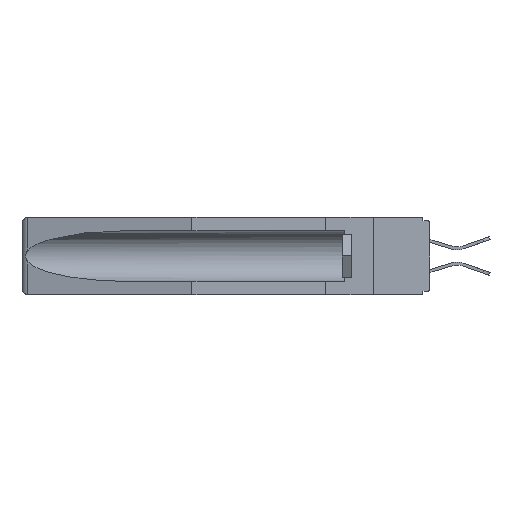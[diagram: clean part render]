
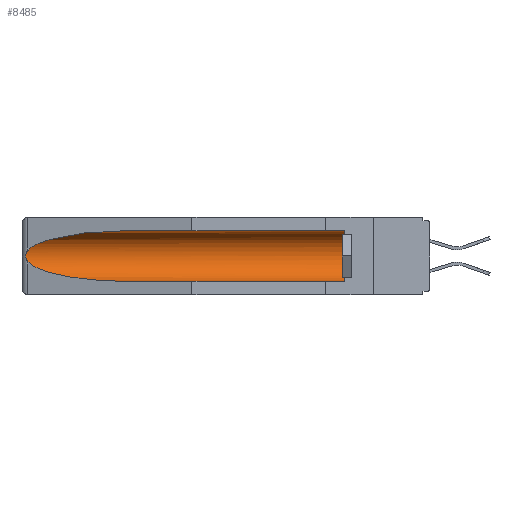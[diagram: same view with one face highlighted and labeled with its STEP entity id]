
A CAD part, left-side view. The second image highlights one B-rep face of the part: STEP entity #8485.
In plain terms, the highlighted cylindrical face has radius 2.857 mm (diameter 5.715 mm), a partial arc.
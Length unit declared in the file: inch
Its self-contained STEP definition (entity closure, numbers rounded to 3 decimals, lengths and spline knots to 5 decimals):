
#535 = AXIS2_PLACEMENT_3D ( 'NONE', #24284, #26498, #13403 ) ;
#593 = EDGE_CURVE ( 'NONE', #28294, #17367, #24356, .T. ) ;
#643 = EDGE_CURVE ( 'NONE', #16500, #28294, #3115, .T. ) ;
#1154 = CARTESIAN_POINT ( 'NONE',  ( 0.26537, 1.52718, -0.19328 ) ) ;
#2209 = CARTESIAN_POINT ( 'NONE',  ( 0.155, 1.07973, -0.059 ) ) ;
#3101 = VERTEX_POINT ( 'NONE', #14312 ) ;
#3115 = B_SPLINE_CURVE_WITH_KNOTS ( 'NONE', 3,
 ( #3253, #23229, #25435, #16695, #3615, #5355, #20636, #7530, #18514, #22962 ),
 .UNSPECIFIED., .F., .F.,
 ( 4, 2, 2, 2, 4 ),
 ( 0., 0.00029, 0.00058, 0.00087, 0.00117 ),
 .UNSPECIFIED. ) ;
#3253 = CARTESIAN_POINT ( 'NONE',  ( 0.26537, 1.52718, -0.14972 ) ) ;
#3615 = CARTESIAN_POINT ( 'NONE',  ( 0.2675, 1.53308, -0.16763 ) ) ;
#3891 = VERTEX_POINT ( 'NONE', #6112 ) ;
#5323 = AXIS2_PLACEMENT_3D ( 'NONE', #17474, #10945, #17375 ) ;
#5355 = CARTESIAN_POINT ( 'NONE',  ( 0.2675, 1.53308, -0.17534 ) ) ;
#5630 = CARTESIAN_POINT ( 'NONE',  ( 0.25451, 1.48313, -0.24835 ) ) ;
#6112 = CARTESIAN_POINT ( 'NONE',  ( 0.155, 1.07973, -0.059 ) ) ;
#6409 = ORIENTED_EDGE ( 'NONE', *, *, #643, .T. ) ;
#7530 = CARTESIAN_POINT ( 'NONE',  ( 0.26655, 1.53094, -0.18657 ) ) ;
#7807 = CARTESIAN_POINT ( 'NONE',  ( 0.21114, 1.30732, -0.284 ) ) ;
#7899 = CARTESIAN_POINT ( 'NONE',  ( 0.155, 1.07973, -0.284 ) ) ;
#8485 = ADVANCED_FACE ( 'NONE', ( #27992 ), #13875, .F. ) ;
#9525 = DIRECTION ( 'NONE',  ( 0., 1., 0. ) ) ;
#9707 = CARTESIAN_POINT ( 'NONE',  ( 0.26537, 1.52718, -0.14972 ) ) ;
#10874 = CARTESIAN_POINT ( 'NONE',  ( 0.155, 1.07973, -0.284 ) ) ;
#10945 = DIRECTION ( 'NONE',  ( 0., -1., 0. ) ) ;
#11147 =( BOUNDED_CURVE ( )  B_SPLINE_CURVE ( 3, ( #2209, #15069, #26049, #21698 ),
 .UNSPECIFIED., .F., .F. ) 
 B_SPLINE_CURVE_WITH_KNOTS ( ( 4, 4 ),
 ( 4.71239, 6.08839 ),
 .UNSPECIFIED. ) 
 CURVE ( )  GEOMETRIC_REPRESENTATION_ITEM ( )  RATIONAL_B_SPLINE_CURVE ( ( 1., 0.848, 0.848, 1. ) ) 
 REPRESENTATION_ITEM ( '' )  );
#11798 = DIRECTION ( 'NONE',  ( 0., 1., 0. ) ) ;
#13403 = DIRECTION ( 'NONE',  ( 0., 0., 1. ) ) ;
#13875 = CYLINDRICAL_SURFACE ( 'NONE', #535, 0.1125 ) ;
#14205 = EDGE_LOOP ( 'NONE', ( #18307, #6409, #16696, #26466, #26667, #27182 ) ) ;
#14312 = CARTESIAN_POINT ( 'NONE',  ( 0.155, 0.126, -0.284 ) ) ;
#15069 = CARTESIAN_POINT ( 'NONE',  ( 0.21114, 1.30732, -0.059 ) ) ;
#15825 = CARTESIAN_POINT ( 'NONE',  ( 0.155, -0.30754, -0.059 ) ) ;
#16500 = VERTEX_POINT ( 'NONE', #9707 ) ;
#16695 = CARTESIAN_POINT ( 'NONE',  ( 0.2673, 1.5327, -0.16383 ) ) ;
#16696 = ORIENTED_EDGE ( 'NONE', *, *, #593, .T. ) ;
#17347 = EDGE_CURVE ( 'NONE', #3891, #16500, #11147, .T. ) ;
#17367 = VERTEX_POINT ( 'NONE', #10874 ) ;
#17375 = DIRECTION ( 'NONE',  ( 0., 0., 1. ) ) ;
#17474 = CARTESIAN_POINT ( 'NONE',  ( 0.155, 0.126, -0.1715 ) ) ;
#17851 = LINE ( 'NONE', #24862, #19914 ) ;
#18307 = ORIENTED_EDGE ( 'NONE', *, *, #17347, .T. ) ;
#18514 = CARTESIAN_POINT ( 'NONE',  ( 0.26597, 1.5296, -0.19026 ) ) ;
#19023 = LINE ( 'NONE', #15825, #20402 ) ;
#19284 = CARTESIAN_POINT ( 'NONE',  ( 0.155, 0.126, -0.059 ) ) ;
#19914 = VECTOR ( 'NONE', #11798, 39.37008 ) ;
#20402 = VECTOR ( 'NONE', #9525, 39.37008 ) ;
#20436 = CARTESIAN_POINT ( 'NONE',  ( 0.26537, 1.52718, -0.19328 ) ) ;
#20636 = CARTESIAN_POINT ( 'NONE',  ( 0.2673, 1.53269, -0.17917 ) ) ;
#21258 = CIRCLE ( 'NONE', #5323, 0.1125 ) ;
#21698 = CARTESIAN_POINT ( 'NONE',  ( 0.26537, 1.52718, -0.14972 ) ) ;
#22962 = CARTESIAN_POINT ( 'NONE',  ( 0.26537, 1.52718, -0.19328 ) ) ;
#23229 = CARTESIAN_POINT ( 'NONE',  ( 0.26597, 1.52961, -0.15275 ) ) ;
#23239 = EDGE_CURVE ( 'NONE', #3101, #26642, #21258, .T. ) ;
#23590 = EDGE_CURVE ( 'NONE', #3101, #17367, #17851, .T. ) ;
#24284 = CARTESIAN_POINT ( 'NONE',  ( 0.155, -0.30754, -0.1715 ) ) ;
#24356 =( BOUNDED_CURVE ( )  B_SPLINE_CURVE ( 3, ( #1154, #5630, #7807, #7899 ),
 .UNSPECIFIED., .F., .F. ) 
 B_SPLINE_CURVE_WITH_KNOTS ( ( 4, 4 ),
 ( 0.1948, 1.5708 ),
 .UNSPECIFIED. ) 
 CURVE ( )  GEOMETRIC_REPRESENTATION_ITEM ( )  RATIONAL_B_SPLINE_CURVE ( ( 1., 0.848, 0.848, 1. ) ) 
 REPRESENTATION_ITEM ( '' )  );
#24862 = CARTESIAN_POINT ( 'NONE',  ( 0.155, -0.30754, -0.284 ) ) ;
#25435 = CARTESIAN_POINT ( 'NONE',  ( 0.26654, 1.53092, -0.15636 ) ) ;
#26049 = CARTESIAN_POINT ( 'NONE',  ( 0.25451, 1.48313, -0.09465 ) ) ;
#26466 = ORIENTED_EDGE ( 'NONE', *, *, #23590, .F. ) ;
#26498 = DIRECTION ( 'NONE',  ( 0., 1., 0. ) ) ;
#26642 = VERTEX_POINT ( 'NONE', #19284 ) ;
#26667 = ORIENTED_EDGE ( 'NONE', *, *, #23239, .T. ) ;
#26684 = EDGE_CURVE ( 'NONE', #26642, #3891, #19023, .T. ) ;
#27182 = ORIENTED_EDGE ( 'NONE', *, *, #26684, .T. ) ;
#27992 = FACE_OUTER_BOUND ( 'NONE', #14205, .T. ) ;
#28294 = VERTEX_POINT ( 'NONE', #20436 ) ;
